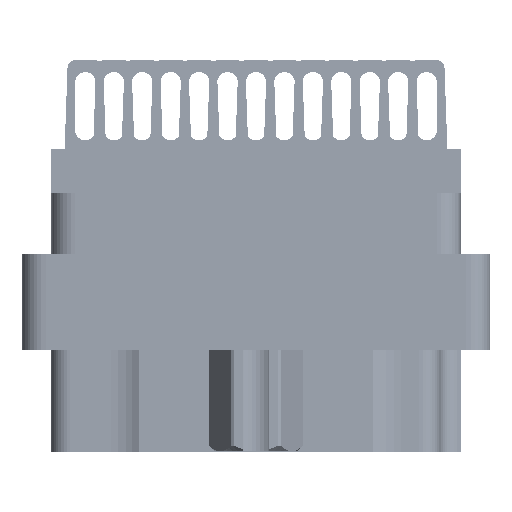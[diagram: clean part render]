
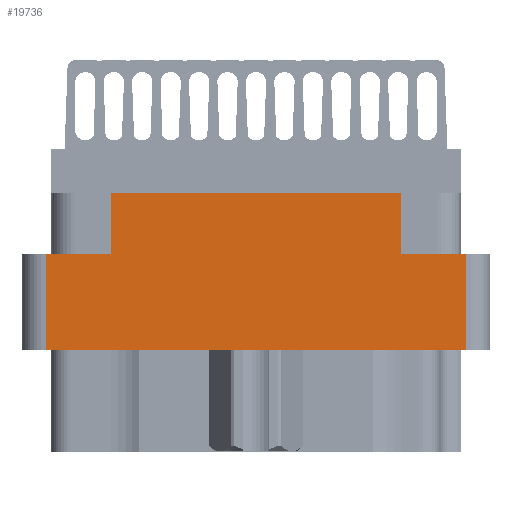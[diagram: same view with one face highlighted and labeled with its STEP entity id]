
A CAD part, left-side view. The second image highlights one B-rep face of the part: STEP entity #19736.
In plain terms, the highlighted planar face has unit normal (-1, 0, 0).
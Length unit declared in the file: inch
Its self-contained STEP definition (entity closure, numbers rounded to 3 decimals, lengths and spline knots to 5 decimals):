
#3149 = EDGE_CURVE ( 'NONE', #7228, #9878, #49670, .T. ) ;
#3665 = CARTESIAN_POINT ( 'NONE',  ( -1.359, -0.617, -0.798 ) ) ;
#6266 = DIRECTION ( 'NONE',  ( 0., 1., 0. ) ) ;
#6431 = ORIENTED_EDGE ( 'NONE', *, *, #13797, .T. ) ;
#7228 = VERTEX_POINT ( 'NONE', #35761 ) ;
#8091 = LINE ( 'NONE', #39582, #26341 ) ;
#9448 = ORIENTED_EDGE ( 'NONE', *, *, #14436, .F. ) ;
#9878 = VERTEX_POINT ( 'NONE', #44776 ) ;
#10416 = VERTEX_POINT ( 'NONE', #61886 ) ;
#10634 = CARTESIAN_POINT ( 'NONE',  ( -1.359, -0.555, -0.529 ) ) ;
#10769 = EDGE_CURVE ( 'NONE', #10416, #30096, #37989, .T. ) ;
#13797 = EDGE_CURVE ( 'NONE', #70266, #30096, #8091, .T. ) ;
#13840 = DIRECTION ( 'NONE',  ( 0., 0., 1. ) ) ;
#14436 = EDGE_CURVE ( 'NONE', #53882, #10416, #16085, .T. ) ;
#15575 = DIRECTION ( 'NONE',  ( 0., 0., 1. ) ) ;
#16085 = LINE ( 'NONE', #80414, #68736 ) ;
#16804 = CARTESIAN_POINT ( 'NONE',  ( -1.359, 0., -0.277 ) ) ;
#18978 = CARTESIAN_POINT ( 'NONE',  ( -1.359, 0., -0.529 ) ) ;
#19372 = LINE ( 'NONE', #82935, #61948 ) ;
#19428 = ORIENTED_EDGE ( 'NONE', *, *, #61394, .F. ) ;
#19478 = ORIENTED_EDGE ( 'NONE', *, *, #54282, .F. ) ;
#19594 = EDGE_CURVE ( 'NONE', #70266, #70444, #19372, .T. ) ;
#19736 = ADVANCED_FACE ( 'NONE', ( #29536 ), #22606, .T. ) ;
#22606 = PLANE ( 'NONE',  #49555 ) ;
#24759 = CARTESIAN_POINT ( 'NONE',  ( -1.359, -0.555, -0.277 ) ) ;
#25410 = ORIENTED_EDGE ( 'NONE', *, *, #10769, .F. ) ;
#26341 = VECTOR ( 'NONE', #13840, 39.37008 ) ;
#27575 = CARTESIAN_POINT ( 'NONE',  ( -1.359, 0.617, -0.117 ) ) ;
#29536 = FACE_OUTER_BOUND ( 'NONE', #36033, .T. ) ;
#29786 = DIRECTION ( 'NONE',  ( 0., 0., 1. ) ) ;
#30096 = VERTEX_POINT ( 'NONE', #82842 ) ;
#30392 = ORIENTED_EDGE ( 'NONE', *, *, #19594, .F. ) ;
#30874 = VECTOR ( 'NONE', #73658, 39.37008 ) ;
#35761 = CARTESIAN_POINT ( 'NONE',  ( -1.359, 0.555, -0.277 ) ) ;
#36033 = EDGE_LOOP ( 'NONE', ( #19478, #64933, #19428, #47140, #30392, #6431, #25410, #9448 ) ) ;
#36564 = VECTOR ( 'NONE', #69611, 39.37008 ) ;
#37094 = CARTESIAN_POINT ( 'NONE',  ( -1.359, 0.555, -0.798 ) ) ;
#37989 = LINE ( 'NONE', #27575, #30874 ) ;
#38943 = VECTOR ( 'NONE', #41395, 39.37008 ) ;
#39582 = CARTESIAN_POINT ( 'NONE',  ( -1.359, -0.3825, -0.277 ) ) ;
#40320 = VECTOR ( 'NONE', #82715, 39.37008 ) ;
#41395 = DIRECTION ( 'NONE',  ( 0., 0., 1. ) ) ;
#42338 = CARTESIAN_POINT ( 'NONE',  ( -1.359, -0.3825, -0.277 ) ) ;
#44776 = CARTESIAN_POINT ( 'NONE',  ( -1.359, 0.555, -0.529 ) ) ;
#45139 = CARTESIAN_POINT ( 'NONE',  ( -1.359, 0.3825, -0.277 ) ) ;
#47140 = ORIENTED_EDGE ( 'NONE', *, *, #82410, .T. ) ;
#49555 = AXIS2_PLACEMENT_3D ( 'NONE', #3665, #67900, #15575 ) ;
#49670 = LINE ( 'NONE', #37094, #36564 ) ;
#49717 = LINE ( 'NONE', #18978, #81114 ) ;
#53882 = VERTEX_POINT ( 'NONE', #45139 ) ;
#54282 = EDGE_CURVE ( 'NONE', #7228, #53882, #61568, .T. ) ;
#61394 = EDGE_CURVE ( 'NONE', #76694, #9878, #49717, .T. ) ;
#61568 = LINE ( 'NONE', #16804, #40320 ) ;
#61886 = CARTESIAN_POINT ( 'NONE',  ( -1.359, 0.3825, -0.117 ) ) ;
#61948 = VECTOR ( 'NONE', #63705, 39.37008 ) ;
#63705 = DIRECTION ( 'NONE',  ( 0., -1., 0. ) ) ;
#64933 = ORIENTED_EDGE ( 'NONE', *, *, #3149, .T. ) ;
#67900 = DIRECTION ( 'NONE',  ( -1., 0., 0. ) ) ;
#68736 = VECTOR ( 'NONE', #29786, 39.37008 ) ;
#69611 = DIRECTION ( 'NONE',  ( 0., 0., -1. ) ) ;
#70266 = VERTEX_POINT ( 'NONE', #42338 ) ;
#70444 = VERTEX_POINT ( 'NONE', #24759 ) ;
#73356 = LINE ( 'NONE', #80385, #38943 ) ;
#73658 = DIRECTION ( 'NONE',  ( 0., -1., 0. ) ) ;
#76694 = VERTEX_POINT ( 'NONE', #10634 ) ;
#80385 = CARTESIAN_POINT ( 'NONE',  ( -1.359, -0.555, -0.798 ) ) ;
#80414 = CARTESIAN_POINT ( 'NONE',  ( -1.359, 0.3825, -0.277 ) ) ;
#81114 = VECTOR ( 'NONE', #6266, 39.37008 ) ;
#82410 = EDGE_CURVE ( 'NONE', #76694, #70444, #73356, .T. ) ;
#82715 = DIRECTION ( 'NONE',  ( 0., -1., 0. ) ) ;
#82842 = CARTESIAN_POINT ( 'NONE',  ( -1.359, -0.3825, -0.117 ) ) ;
#82935 = CARTESIAN_POINT ( 'NONE',  ( -1.359, 0., -0.277 ) ) ;
